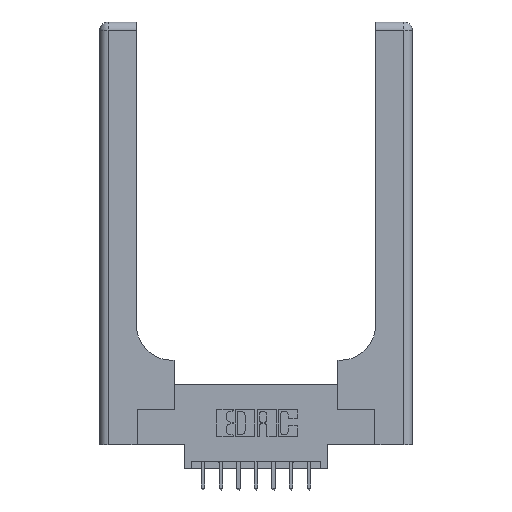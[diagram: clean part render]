
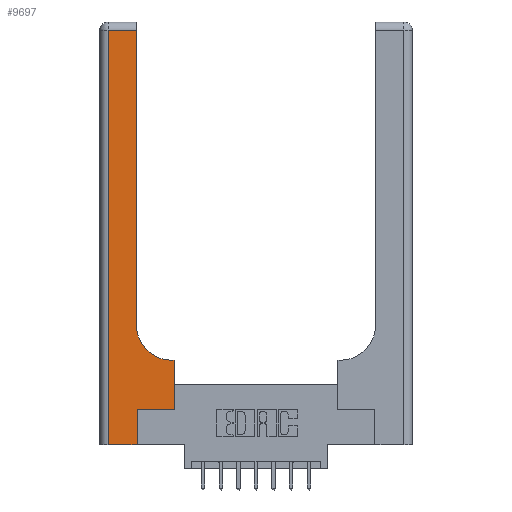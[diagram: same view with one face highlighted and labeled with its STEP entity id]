
A CAD part, top view. The second image highlights one B-rep face of the part: STEP entity #9697.
In plain terms, the highlighted planar face has unit normal (0, 0, 1).
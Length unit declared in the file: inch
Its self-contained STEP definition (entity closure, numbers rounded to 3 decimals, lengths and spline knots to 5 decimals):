
#224 = EDGE_CURVE ( 'NONE', #6184, #4183, #4988, .T. ) ;
#258 = FACE_OUTER_BOUND ( 'NONE', #12733, .T. ) ;
#444 = CARTESIAN_POINT ( 'NONE',  ( 0.06, 3., 0.37 ) ) ;
#499 = CARTESIAN_POINT ( 'NONE',  ( 0.51, 0.6, 0.37 ) ) ;
#541 = ORIENTED_EDGE ( 'NONE', *, *, #5105, .T. ) ;
#973 = EDGE_CURVE ( 'NONE', #5106, #12374, #11038, .T. ) ;
#1177 = VERTEX_POINT ( 'NONE', #10491 ) ;
#1408 = CARTESIAN_POINT ( 'NONE',  ( 0.26, 3., 0.37 ) ) ;
#1843 = CARTESIAN_POINT ( 'NONE',  ( 0.528, 0.6, 0.37 ) ) ;
#1880 = EDGE_CURVE ( 'NONE', #6648, #14799, #4014, .T. ) ;
#2298 = LINE ( 'NONE', #13677, #4304 ) ;
#2365 = VECTOR ( 'NONE', #13081, 39.37008 ) ;
#2374 = CARTESIAN_POINT ( 'NONE',  ( 0., 3., 0.37 ) ) ;
#2570 = ORIENTED_EDGE ( 'NONE', *, *, #14311, .T. ) ;
#2737 = CARTESIAN_POINT ( 'NONE',  ( 0.26, 0.85, 0.37 ) ) ;
#3385 = CARTESIAN_POINT ( 'NONE',  ( 0.26, 0.6, 0.37 ) ) ;
#3663 = DIRECTION ( 'NONE',  ( 0., -1., 0. ) ) ;
#3760 = DIRECTION ( 'NONE',  ( 0., 1., 0. ) ) ;
#3785 = VECTOR ( 'NONE', #9319, 39.37008 ) ;
#3816 = CARTESIAN_POINT ( 'NONE',  ( 0.265, 0.25, 0.37 ) ) ;
#3852 = CARTESIAN_POINT ( 'NONE',  ( 0.51, 0.85, 0.37 ) ) ;
#4014 = LINE ( 'NONE', #8677, #8556 ) ;
#4084 = EDGE_CURVE ( 'NONE', #1177, #5106, #14123, .T. ) ;
#4183 = VERTEX_POINT ( 'NONE', #3816 ) ;
#4304 = VECTOR ( 'NONE', #5742, 39.37008 ) ;
#4966 = ORIENTED_EDGE ( 'NONE', *, *, #9093, .T. ) ;
#4988 = LINE ( 'NONE', #8506, #2365 ) ;
#5105 = EDGE_CURVE ( 'NONE', #6168, #1177, #14214, .T. ) ;
#5106 = VERTEX_POINT ( 'NONE', #8278 ) ;
#5323 = VECTOR ( 'NONE', #13806, 39.37008 ) ;
#5331 = VERTEX_POINT ( 'NONE', #499 ) ;
#5742 = DIRECTION ( 'NONE',  ( 1., 0., 0. ) ) ;
#6168 = VERTEX_POINT ( 'NONE', #2737 ) ;
#6184 = VERTEX_POINT ( 'NONE', #10896 ) ;
#6479 = ORIENTED_EDGE ( 'NONE', *, *, #10755, .T. ) ;
#6559 = AXIS2_PLACEMENT_3D ( 'NONE', #3852, #9730, #12168 ) ;
#6648 = VERTEX_POINT ( 'NONE', #7910 ) ;
#6952 = CARTESIAN_POINT ( 'NONE',  ( 0.06, 0., 0.37 ) ) ;
#7752 = ORIENTED_EDGE ( 'NONE', *, *, #973, .T. ) ;
#7910 = CARTESIAN_POINT ( 'NONE',  ( 0.528, 0.25, 0.37 ) ) ;
#8274 = VECTOR ( 'NONE', #13985, 39.37008 ) ;
#8278 = CARTESIAN_POINT ( 'NONE',  ( 0.06, 2.94, 0.37 ) ) ;
#8481 = DIRECTION ( 'NONE',  ( -1., 0., 0. ) ) ;
#8506 = CARTESIAN_POINT ( 'NONE',  ( 0.265, 0., 0.37 ) ) ;
#8556 = VECTOR ( 'NONE', #13332, 39.37008 ) ;
#8677 = CARTESIAN_POINT ( 'NONE',  ( 0.528, 0.25, 0.37 ) ) ;
#9086 = CARTESIAN_POINT ( 'NONE',  ( 0.265, 0.25, 0.37 ) ) ;
#9093 = EDGE_CURVE ( 'NONE', #14799, #5331, #9266, .T. ) ;
#9119 = ORIENTED_EDGE ( 'NONE', *, *, #1880, .T. ) ;
#9266 = LINE ( 'NONE', #3385, #8274 ) ;
#9319 = DIRECTION ( 'NONE',  ( -1., 0., 0. ) ) ;
#9457 = ORIENTED_EDGE ( 'NONE', *, *, #4084, .T. ) ;
#9535 = ORIENTED_EDGE ( 'NONE', *, *, #224, .T. ) ;
#9697 = ADVANCED_FACE ( 'NONE', ( #258 ), #12913, .F. ) ;
#9710 = CIRCLE ( 'NONE', #6559, 0.25 ) ;
#9730 = DIRECTION ( 'NONE',  ( 0., 0., -1. ) ) ;
#9820 = VECTOR ( 'NONE', #3663, 39.37008 ) ;
#10143 = VECTOR ( 'NONE', #3760, 39.37008 ) ;
#10491 = CARTESIAN_POINT ( 'NONE',  ( 0.26, 2.94, 0.37 ) ) ;
#10755 = EDGE_CURVE ( 'NONE', #12374, #6184, #2298, .T. ) ;
#10896 = CARTESIAN_POINT ( 'NONE',  ( 0.265, 0., 0.37 ) ) ;
#11038 = LINE ( 'NONE', #444, #9820 ) ;
#11460 = AXIS2_PLACEMENT_3D ( 'NONE', #2374, #11920, #8481 ) ;
#11920 = DIRECTION ( 'NONE',  ( 0., 0., -1. ) ) ;
#12168 = DIRECTION ( 'NONE',  ( 1., 0., 0. ) ) ;
#12374 = VERTEX_POINT ( 'NONE', #6952 ) ;
#12733 = EDGE_LOOP ( 'NONE', ( #541, #9457, #7752, #6479, #9535, #14640, #9119, #4966, #2570 ) ) ;
#12913 = PLANE ( 'NONE',  #11460 ) ;
#12984 = CARTESIAN_POINT ( 'NONE',  ( 0., 2.94, 0.37 ) ) ;
#13081 = DIRECTION ( 'NONE',  ( 0., 1., 0. ) ) ;
#13332 = DIRECTION ( 'NONE',  ( 0., 1., 0. ) ) ;
#13677 = CARTESIAN_POINT ( 'NONE',  ( 0., 0., 0.37 ) ) ;
#13788 = EDGE_CURVE ( 'NONE', #4183, #6648, #14869, .T. ) ;
#13806 = DIRECTION ( 'NONE',  ( 1., 0., 0. ) ) ;
#13985 = DIRECTION ( 'NONE',  ( -1., 0., 0. ) ) ;
#14123 = LINE ( 'NONE', #12984, #3785 ) ;
#14214 = LINE ( 'NONE', #1408, #10143 ) ;
#14311 = EDGE_CURVE ( 'NONE', #5331, #6168, #9710, .T. ) ;
#14640 = ORIENTED_EDGE ( 'NONE', *, *, #13788, .T. ) ;
#14799 = VERTEX_POINT ( 'NONE', #1843 ) ;
#14869 = LINE ( 'NONE', #9086, #5323 ) ;
